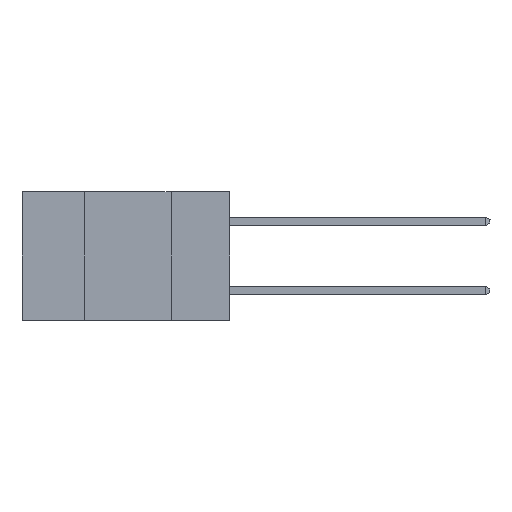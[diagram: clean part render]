
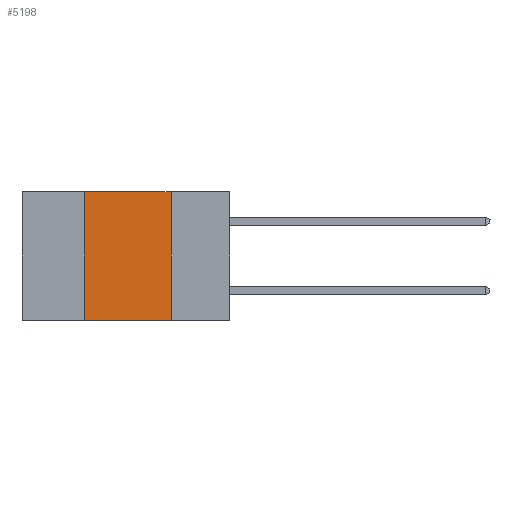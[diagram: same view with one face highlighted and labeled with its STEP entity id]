
A CAD part, left-side view. The second image highlights one B-rep face of the part: STEP entity #5198.
In plain terms, the highlighted planar face has unit normal (-1, 0, 0).
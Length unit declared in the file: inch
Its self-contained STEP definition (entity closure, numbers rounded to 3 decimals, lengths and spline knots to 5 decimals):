
#565 = LINE ( 'NONE', #10246, #22592 ) ;
#1840 = ORIENTED_EDGE ( 'NONE', *, *, #2680, .T. ) ;
#2680 = EDGE_CURVE ( 'NONE', #25218, #14284, #11126, .T. ) ;
#3339 = VERTEX_POINT ( 'NONE', #11930 ) ;
#3383 = DIRECTION ( 'NONE',  ( 0., -1., 0. ) ) ;
#5198 = ADVANCED_FACE ( 'NONE', ( #9986 ), #16298, .F. ) ;
#5413 = VECTOR ( 'NONE', #11667, 39.37008 ) ;
#5724 = DIRECTION ( 'NONE',  ( 0., 0., -1. ) ) ;
#8107 = DIRECTION ( 'NONE',  ( 0., 0., -1. ) ) ;
#9425 = VECTOR ( 'NONE', #3383, 39.37008 ) ;
#9464 = AXIS2_PLACEMENT_3D ( 'NONE', #16388, #18506, #5724 ) ;
#9548 = CARTESIAN_POINT ( 'NONE',  ( 0., 0.6, -0.37 ) ) ;
#9986 = FACE_OUTER_BOUND ( 'NONE', #23950, .T. ) ;
#10246 = CARTESIAN_POINT ( 'NONE',  ( 0., 0.17, 0. ) ) ;
#10333 = CARTESIAN_POINT ( 'NONE',  ( 0., 0.42, 0. ) ) ;
#11126 = LINE ( 'NONE', #9548, #5413 ) ;
#11667 = DIRECTION ( 'NONE',  ( 0., -1., 0. ) ) ;
#11911 = CARTESIAN_POINT ( 'NONE',  ( 0., 0.17, -0.37 ) ) ;
#11930 = CARTESIAN_POINT ( 'NONE',  ( 0., 0.17, 0. ) ) ;
#11952 = ORIENTED_EDGE ( 'NONE', *, *, #15715, .F. ) ;
#12605 = ORIENTED_EDGE ( 'NONE', *, *, #24601, .F. ) ;
#14066 = CARTESIAN_POINT ( 'NONE',  ( 0., 0.6, 0. ) ) ;
#14284 = VERTEX_POINT ( 'NONE', #11911 ) ;
#14934 = CARTESIAN_POINT ( 'NONE',  ( 0., 0.42, -0.37 ) ) ;
#15052 = LINE ( 'NONE', #14066, #9425 ) ;
#15139 = LINE ( 'NONE', #10333, #25619 ) ;
#15715 = EDGE_CURVE ( 'NONE', #21361, #3339, #15052, .T. ) ;
#16298 = PLANE ( 'NONE',  #9464 ) ;
#16388 = CARTESIAN_POINT ( 'NONE',  ( 0., 0.6, 0. ) ) ;
#18506 = DIRECTION ( 'NONE',  ( 1., 0., 0. ) ) ;
#18980 = EDGE_CURVE ( 'NONE', #3339, #14284, #565, .T. ) ;
#21361 = VERTEX_POINT ( 'NONE', #23565 ) ;
#22528 = ORIENTED_EDGE ( 'NONE', *, *, #18980, .F. ) ;
#22592 = VECTOR ( 'NONE', #8107, 39.37008 ) ;
#23565 = CARTESIAN_POINT ( 'NONE',  ( 0., 0.42, 0. ) ) ;
#23950 = EDGE_LOOP ( 'NONE', ( #22528, #11952, #12605, #1840 ) ) ;
#24601 = EDGE_CURVE ( 'NONE', #25218, #21361, #15139, .T. ) ;
#25083 = DIRECTION ( 'NONE',  ( 0., 0., 1. ) ) ;
#25218 = VERTEX_POINT ( 'NONE', #14934 ) ;
#25619 = VECTOR ( 'NONE', #25083, 39.37008 ) ;
